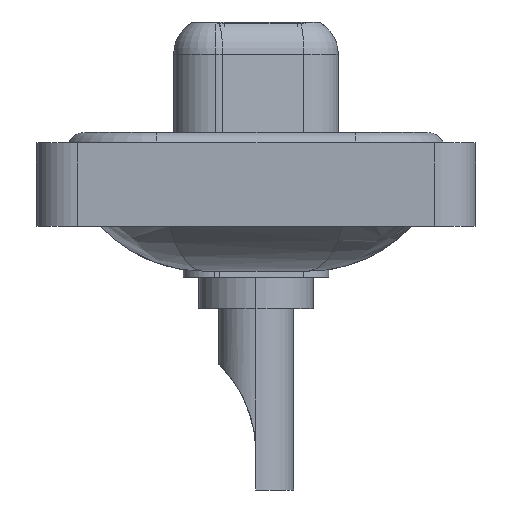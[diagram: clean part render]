
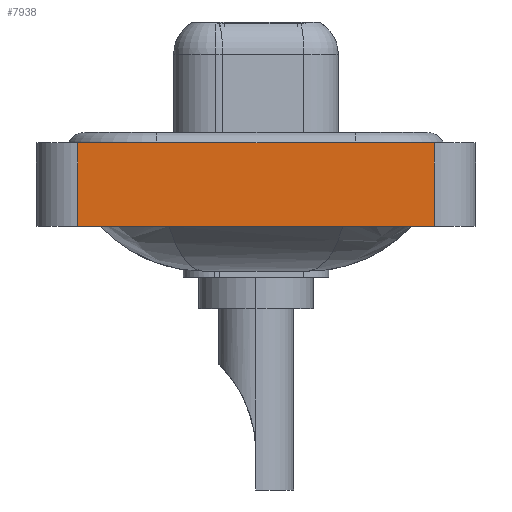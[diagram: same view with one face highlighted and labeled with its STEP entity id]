
A CAD part, left-side view. The second image highlights one B-rep face of the part: STEP entity #7938.
In plain terms, the highlighted planar face has unit normal (-1, 0, 0).
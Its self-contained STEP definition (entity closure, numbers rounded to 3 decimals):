
#34 = DIRECTION ( 'NONE',  ( 0., -1., 0. ) ) ;
#93 = DIRECTION ( 'NONE',  ( 0., 0., 1. ) ) ;
#325 = LINE ( 'NONE', #658, #8855 ) ;
#658 = CARTESIAN_POINT ( 'NONE',  ( -7.35, -8.55, -3.6 ) ) ;
#1201 = CARTESIAN_POINT ( 'NONE',  ( -7.35, 8.55, -3.6 ) ) ;
#2201 = EDGE_CURVE ( 'NONE', #3289, #5092, #15454, .T. ) ;
#2651 = EDGE_LOOP ( 'NONE', ( #13610, #6123, #4672, #15023 ) ) ;
#2849 = VECTOR ( 'NONE', #34, 1000. ) ;
#2920 = DIRECTION ( 'NONE',  ( 0., 0., 1. ) ) ;
#3289 = VERTEX_POINT ( 'NONE', #12003 ) ;
#3595 = EDGE_CURVE ( 'NONE', #10274, #3289, #4126, .T. ) ;
#3959 = DIRECTION ( 'NONE',  ( 0., -1., 0. ) ) ;
#4126 = LINE ( 'NONE', #1201, #9393 ) ;
#4672 = ORIENTED_EDGE ( 'NONE', *, *, #3595, .F. ) ;
#4897 = DIRECTION ( 'NONE',  ( 0., 0., 1. ) ) ;
#5092 = VERTEX_POINT ( 'NONE', #5466 ) ;
#5312 = LINE ( 'NONE', #9257, #2849 ) ;
#5466 = CARTESIAN_POINT ( 'NONE',  ( -7.35, -8.55, 0.4 ) ) ;
#6123 = ORIENTED_EDGE ( 'NONE', *, *, #2201, .F. ) ;
#6238 = CARTESIAN_POINT ( 'NONE',  ( -7.35, -8.55, -3.6 ) ) ;
#7938 = ADVANCED_FACE ( 'NONE', ( #15131 ), #13798, .T. ) ;
#8632 = CARTESIAN_POINT ( 'NONE',  ( -7.35, -8.55, -3.6 ) ) ;
#8663 = AXIS2_PLACEMENT_3D ( 'NONE', #6238, #16560, #4897 ) ;
#8855 = VECTOR ( 'NONE', #2920, 1000. ) ;
#8985 = VERTEX_POINT ( 'NONE', #8632 ) ;
#9257 = CARTESIAN_POINT ( 'NONE',  ( -7.35, -8.55, -3.6 ) ) ;
#9393 = VECTOR ( 'NONE', #93, 1000. ) ;
#10143 = CARTESIAN_POINT ( 'NONE',  ( -7.35, 8.55, -3.6 ) ) ;
#10274 = VERTEX_POINT ( 'NONE', #10143 ) ;
#10810 = EDGE_CURVE ( 'NONE', #10274, #8985, #5312, .T. ) ;
#10853 = VECTOR ( 'NONE', #3959, 1000. ) ;
#12003 = CARTESIAN_POINT ( 'NONE',  ( -7.35, 8.55, 0.4 ) ) ;
#13069 = EDGE_CURVE ( 'NONE', #8985, #5092, #325, .T. ) ;
#13610 = ORIENTED_EDGE ( 'NONE', *, *, #13069, .T. ) ;
#13798 = PLANE ( 'NONE',  #8663 ) ;
#14274 = CARTESIAN_POINT ( 'NONE',  ( -7.35, -8.55, 0.4 ) ) ;
#15023 = ORIENTED_EDGE ( 'NONE', *, *, #10810, .T. ) ;
#15131 = FACE_OUTER_BOUND ( 'NONE', #2651, .T. ) ;
#15454 = LINE ( 'NONE', #14274, #10853 ) ;
#16560 = DIRECTION ( 'NONE',  ( -1., 0., 0. ) ) ;
